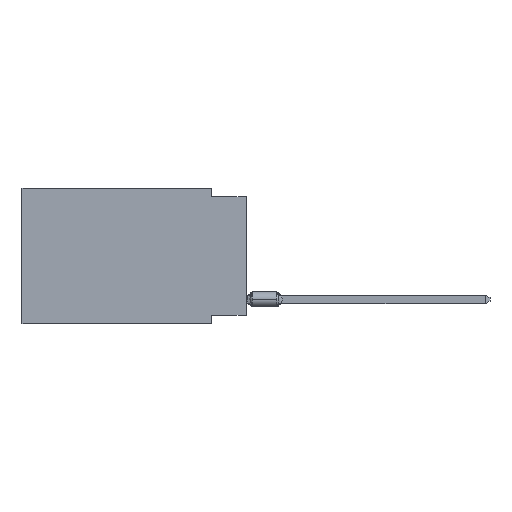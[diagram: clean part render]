
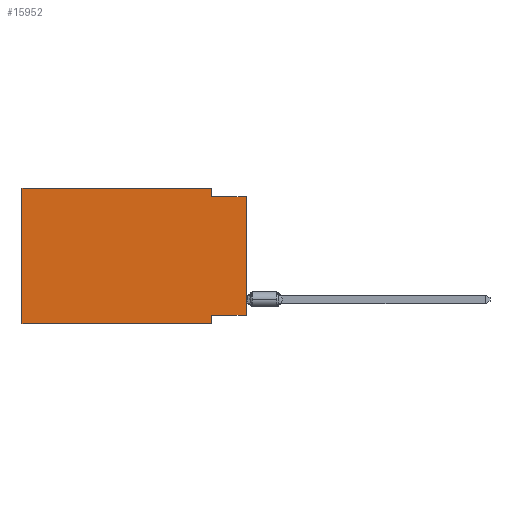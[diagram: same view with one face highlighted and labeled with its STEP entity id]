
A CAD part, left-side view. The second image highlights one B-rep face of the part: STEP entity #15952.
In plain terms, the highlighted planar face has unit normal (-1, 0, 0).
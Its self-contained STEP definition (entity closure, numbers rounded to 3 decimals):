
#771 = CARTESIAN_POINT ( 'NONE',  ( 0., 0., 0. ) ) ;
#1375 = LINE ( 'NONE', #12750, #22594 ) ;
#1837 = LINE ( 'NONE', #13387, #14121 ) ;
#2004 = DIRECTION ( 'NONE',  ( 1., 0., 0. ) ) ;
#3428 = CARTESIAN_POINT ( 'NONE',  ( 0., 2.54, 0. ) ) ;
#3474 = PLANE ( 'NONE',  #27358 ) ;
#4008 = EDGE_CURVE ( 'NONE', #11516, #8177, #1375, .T. ) ;
#5212 = CARTESIAN_POINT ( 'NONE',  ( 0., 2.54, -9.906 ) ) ;
#5598 = ORIENTED_EDGE ( 'NONE', *, *, #26101, .T. ) ;
#6652 = LINE ( 'NONE', #771, #35945 ) ;
#7240 = DIRECTION ( 'NONE',  ( 0., 0., -1. ) ) ;
#7474 = CARTESIAN_POINT ( 'NONE',  ( 0., 2.54, 0. ) ) ;
#7496 = DIRECTION ( 'NONE',  ( 0., -1., 0. ) ) ;
#8177 = VERTEX_POINT ( 'NONE', #5212 ) ;
#8518 = ORIENTED_EDGE ( 'NONE', *, *, #11623, .F. ) ;
#9676 = DIRECTION ( 'NONE',  ( 0., 1., 0. ) ) ;
#10348 = LINE ( 'NONE', #21888, #22496 ) ;
#10739 = DIRECTION ( 'NONE',  ( 0., -1., 0. ) ) ;
#11516 = VERTEX_POINT ( 'NONE', #28885 ) ;
#11623 = EDGE_CURVE ( 'NONE', #18253, #21784, #14502, .T. ) ;
#12375 = VERTEX_POINT ( 'NONE', #28897 ) ;
#12477 = ORIENTED_EDGE ( 'NONE', *, *, #29860, .F. ) ;
#12750 = CARTESIAN_POINT ( 'NONE',  ( 0., 2.54, -9.906 ) ) ;
#13387 = CARTESIAN_POINT ( 'NONE',  ( 0., 0., -0.635 ) ) ;
#13744 = VECTOR ( 'NONE', #33782, 1000. ) ;
#14121 = VECTOR ( 'NONE', #10739, 1000. ) ;
#14502 = LINE ( 'NONE', #17137, #36379 ) ;
#14761 = CARTESIAN_POINT ( 'NONE',  ( 0., 0., -0.635 ) ) ;
#14874 = VECTOR ( 'NONE', #36464, 1000. ) ;
#15230 = VERTEX_POINT ( 'NONE', #22064 ) ;
#15305 = EDGE_CURVE ( 'NONE', #21784, #21737, #10348, .T. ) ;
#15563 = EDGE_LOOP ( 'NONE', ( #19397, #20064, #24657, #21949, #8518, #5598, #26715, #12477 ) ) ;
#15952 = ADVANCED_FACE ( 'NONE', ( #29403 ), #3474, .F. ) ;
#16720 = VECTOR ( 'NONE', #9676, 1000. ) ;
#17137 = CARTESIAN_POINT ( 'NONE',  ( 0., 16.383, 0. ) ) ;
#18253 = VERTEX_POINT ( 'NONE', #37352 ) ;
#19397 = ORIENTED_EDGE ( 'NONE', *, *, #21742, .T. ) ;
#19976 = DIRECTION ( 'NONE',  ( 0., 0., 1. ) ) ;
#20064 = ORIENTED_EDGE ( 'NONE', *, *, #23441, .F. ) ;
#21737 = VERTEX_POINT ( 'NONE', #3428 ) ;
#21742 = EDGE_CURVE ( 'NONE', #12375, #31301, #6652, .T. ) ;
#21784 = VERTEX_POINT ( 'NONE', #22846 ) ;
#21888 = CARTESIAN_POINT ( 'NONE',  ( 0., 16.383, 0. ) ) ;
#21949 = ORIENTED_EDGE ( 'NONE', *, *, #15305, .F. ) ;
#22064 = CARTESIAN_POINT ( 'NONE',  ( 0., 2.54, -0.635 ) ) ;
#22230 = LINE ( 'NONE', #7474, #13744 ) ;
#22496 = VECTOR ( 'NONE', #7496, 1000. ) ;
#22594 = VECTOR ( 'NONE', #7240, 1000. ) ;
#22646 = LINE ( 'NONE', #36848, #14874 ) ;
#22846 = CARTESIAN_POINT ( 'NONE',  ( 0., 16.383, 0. ) ) ;
#23441 = EDGE_CURVE ( 'NONE', #15230, #31301, #1837, .T. ) ;
#24062 = LINE ( 'NONE', #35612, #16720 ) ;
#24657 = ORIENTED_EDGE ( 'NONE', *, *, #24994, .F. ) ;
#24994 = EDGE_CURVE ( 'NONE', #21737, #15230, #22230, .T. ) ;
#26101 = EDGE_CURVE ( 'NONE', #18253, #8177, #22646, .T. ) ;
#26553 = CARTESIAN_POINT ( 'NONE',  ( 0., 16.383, 0. ) ) ;
#26715 = ORIENTED_EDGE ( 'NONE', *, *, #4008, .F. ) ;
#27358 = AXIS2_PLACEMENT_3D ( 'NONE', #26553, #2004, #30408 ) ;
#28885 = CARTESIAN_POINT ( 'NONE',  ( 0., 2.54, -9.271 ) ) ;
#28897 = CARTESIAN_POINT ( 'NONE',  ( 0., 0., -9.271 ) ) ;
#29403 = FACE_OUTER_BOUND ( 'NONE', #15563, .T. ) ;
#29860 = EDGE_CURVE ( 'NONE', #12375, #11516, #24062, .T. ) ;
#30408 = DIRECTION ( 'NONE',  ( 0., 0., -1. ) ) ;
#31301 = VERTEX_POINT ( 'NONE', #14761 ) ;
#33782 = DIRECTION ( 'NONE',  ( 0., 0., -1. ) ) ;
#35612 = CARTESIAN_POINT ( 'NONE',  ( 0., 0., -9.271 ) ) ;
#35945 = VECTOR ( 'NONE', #36466, 1000. ) ;
#36379 = VECTOR ( 'NONE', #19976, 1000. ) ;
#36464 = DIRECTION ( 'NONE',  ( 0., -1., 0. ) ) ;
#36466 = DIRECTION ( 'NONE',  ( 0., 0., 1. ) ) ;
#36848 = CARTESIAN_POINT ( 'NONE',  ( 0., 16.383, -9.906 ) ) ;
#37352 = CARTESIAN_POINT ( 'NONE',  ( 0., 16.383, -9.906 ) ) ;
